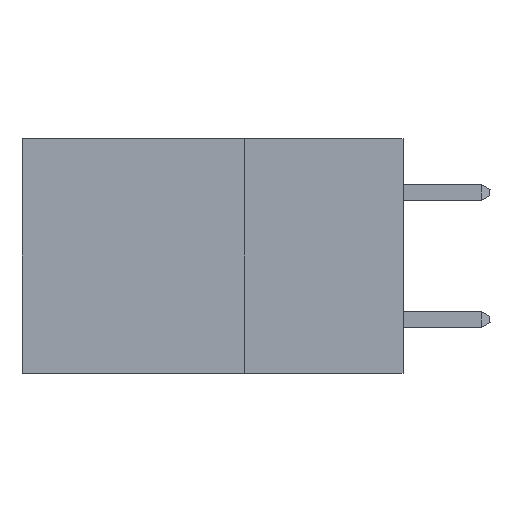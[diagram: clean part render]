
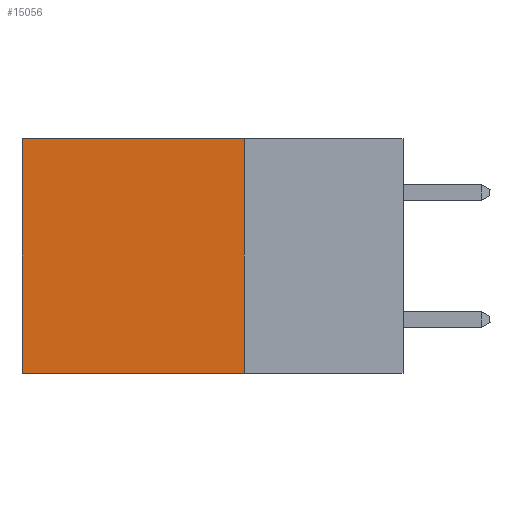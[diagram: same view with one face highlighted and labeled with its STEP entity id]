
A CAD part, left-side view. The second image highlights one B-rep face of the part: STEP entity #15056.
In plain terms, the highlighted planar face has unit normal (-1, 0, 0).
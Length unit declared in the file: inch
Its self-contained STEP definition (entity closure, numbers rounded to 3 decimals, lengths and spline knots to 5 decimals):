
#1102 = EDGE_CURVE ( 'NONE', #13682, #3039, #24338, .T. ) ;
#3039 = VERTEX_POINT ( 'NONE', #27234 ) ;
#3260 = CARTESIAN_POINT ( 'NONE',  ( 0.2875, 0.25, 0. ) ) ;
#3880 = EDGE_CURVE ( 'NONE', #17010, #13682, #29006, .T. ) ;
#4773 = ORIENTED_EDGE ( 'NONE', *, *, #3880, .T. ) ;
#8559 = ORIENTED_EDGE ( 'NONE', *, *, #1102, .T. ) ;
#8649 = CARTESIAN_POINT ( 'NONE',  ( 0.2875, 0.25, 0. ) ) ;
#8764 = CARTESIAN_POINT ( 'NONE',  ( 0.2875, 0.25, 0. ) ) ;
#9389 = ORIENTED_EDGE ( 'NONE', *, *, #21788, .F. ) ;
#11663 = DIRECTION ( 'NONE',  ( 0., 0., -1. ) ) ;
#13682 = VERTEX_POINT ( 'NONE', #15694 ) ;
#15056 = ADVANCED_FACE ( 'NONE', ( #19242 ), #25585, .F. ) ;
#15694 = CARTESIAN_POINT ( 'NONE',  ( 0.2875, 0.6, 0. ) ) ;
#15762 = EDGE_CURVE ( 'NONE', #26920, #3039, #18739, .T. ) ;
#16833 = VECTOR ( 'NONE', #34060, 39.37008 ) ;
#17010 = VERTEX_POINT ( 'NONE', #8649 ) ;
#18739 = LINE ( 'NONE', #25906, #32843 ) ;
#19242 = FACE_OUTER_BOUND ( 'NONE', #27967, .T. ) ;
#19279 = CARTESIAN_POINT ( 'NONE',  ( 0.2875, 0.25, 0. ) ) ;
#19730 = CARTESIAN_POINT ( 'NONE',  ( 0.2875, 0.25, -0.37 ) ) ;
#21788 = EDGE_CURVE ( 'NONE', #17010, #26920, #24597, .T. ) ;
#23442 = DIRECTION ( 'NONE',  ( 0., 0., -1. ) ) ;
#24338 = LINE ( 'NONE', #34103, #16833 ) ;
#24597 = LINE ( 'NONE', #3260, #31242 ) ;
#25092 = AXIS2_PLACEMENT_3D ( 'NONE', #8764, #28680, #11663 ) ;
#25585 = PLANE ( 'NONE',  #25092 ) ;
#25906 = CARTESIAN_POINT ( 'NONE',  ( 0.2875, 0.25, -0.37 ) ) ;
#26920 = VERTEX_POINT ( 'NONE', #19730 ) ;
#27234 = CARTESIAN_POINT ( 'NONE',  ( 0.2875, 0.6, -0.37 ) ) ;
#27967 = EDGE_LOOP ( 'NONE', ( #8559, #31419, #9389, #4773 ) ) ;
#28680 = DIRECTION ( 'NONE',  ( 1., 0., 0. ) ) ;
#28751 = DIRECTION ( 'NONE',  ( 0., 1., 0. ) ) ;
#29006 = LINE ( 'NONE', #19279, #35579 ) ;
#31242 = VECTOR ( 'NONE', #23442, 39.37008 ) ;
#31419 = ORIENTED_EDGE ( 'NONE', *, *, #15762, .F. ) ;
#32843 = VECTOR ( 'NONE', #28751, 39.37008 ) ;
#34060 = DIRECTION ( 'NONE',  ( 0., 0., -1. ) ) ;
#34103 = CARTESIAN_POINT ( 'NONE',  ( 0.2875, 0.6, 0. ) ) ;
#35579 = VECTOR ( 'NONE', #36133, 39.37008 ) ;
#36133 = DIRECTION ( 'NONE',  ( 0., 1., 0. ) ) ;
